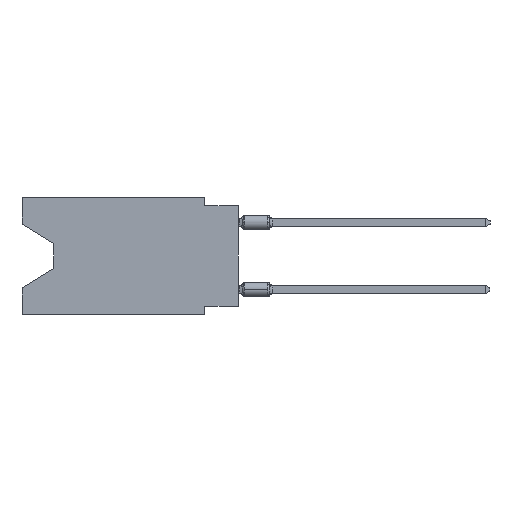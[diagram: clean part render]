
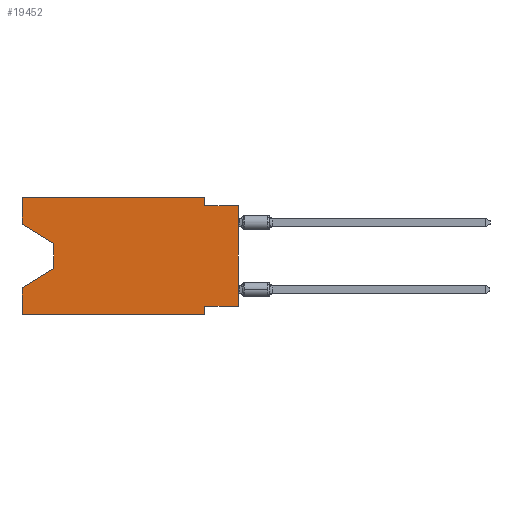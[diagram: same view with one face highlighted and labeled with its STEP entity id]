
A CAD part, left-side view. The second image highlights one B-rep face of the part: STEP entity #19452.
In plain terms, the highlighted planar face has unit normal (-1, 0, 0).
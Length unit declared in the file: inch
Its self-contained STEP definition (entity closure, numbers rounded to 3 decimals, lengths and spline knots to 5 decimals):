
#382 = VERTEX_POINT ( 'NONE', #17225 ) ;
#690 = EDGE_CURVE ( 'NONE', #25854, #382, #19527, .T. ) ;
#716 = CARTESIAN_POINT ( 'NONE',  ( 0., 0., -0.025 ) ) ;
#2037 = VERTEX_POINT ( 'NONE', #716 ) ;
#2414 = VERTEX_POINT ( 'NONE', #17462 ) ;
#3299 = CARTESIAN_POINT ( 'NONE',  ( 0., 0., 0. ) ) ;
#3395 = FACE_OUTER_BOUND ( 'NONE', #7323, .T. ) ;
#3515 = VECTOR ( 'NONE', #14902, 39.37008 ) ;
#3628 = CARTESIAN_POINT ( 'NONE',  ( 0., 0.1, -0.35 ) ) ;
#4466 = EDGE_CURVE ( 'NONE', #28183, #2037, #24819, .T. ) ;
#4566 = EDGE_CURVE ( 'NONE', #10817, #20446, #29086, .T. ) ;
#4943 = EDGE_CURVE ( 'NONE', #7981, #2414, #17398, .T. ) ;
#5505 = EDGE_CURVE ( 'NONE', #20446, #25854, #22928, .T. ) ;
#5774 = VERTEX_POINT ( 'NONE', #11917 ) ;
#6390 = ORIENTED_EDGE ( 'NONE', *, *, #4566, .T. ) ;
#6721 = CARTESIAN_POINT ( 'NONE',  ( 0., 0.645, -0.08025 ) ) ;
#7323 = EDGE_LOOP ( 'NONE', ( #6390, #21658, #12057, #11179, #10332, #13019, #8944, #12033, #10022, #23984, #8794, #13318 ) ) ;
#7707 = DIRECTION ( 'NONE',  ( 0., -1., 0. ) ) ;
#7981 = VERTEX_POINT ( 'NONE', #11597 ) ;
#8347 = LINE ( 'NONE', #3628, #17089 ) ;
#8558 = CARTESIAN_POINT ( 'NONE',  ( 0., 0.645, 0. ) ) ;
#8794 = ORIENTED_EDGE ( 'NONE', *, *, #20240, .F. ) ;
#8944 = ORIENTED_EDGE ( 'NONE', *, *, #9385, .F. ) ;
#9001 = AXIS2_PLACEMENT_3D ( 'NONE', #27774, #13300, #17863 ) ;
#9385 = EDGE_CURVE ( 'NONE', #28183, #25561, #27096, .T. ) ;
#9493 = EDGE_CURVE ( 'NONE', #28814, #5774, #28368, .T. ) ;
#10022 = ORIENTED_EDGE ( 'NONE', *, *, #28672, .F. ) ;
#10083 = DIRECTION ( 'NONE',  ( 0., -0.855, -0.519 ) ) ;
#10332 = ORIENTED_EDGE ( 'NONE', *, *, #9493, .T. ) ;
#10817 = VERTEX_POINT ( 'NONE', #6721 ) ;
#11179 = ORIENTED_EDGE ( 'NONE', *, *, #19741, .F. ) ;
#11256 = CARTESIAN_POINT ( 'NONE',  ( 0., 0.55, -0.212 ) ) ;
#11597 = CARTESIAN_POINT ( 'NONE',  ( 0., 0.1, 0. ) ) ;
#11917 = CARTESIAN_POINT ( 'NONE',  ( 0., 0.1, -0.35 ) ) ;
#12033 = ORIENTED_EDGE ( 'NONE', *, *, #4466, .T. ) ;
#12057 = ORIENTED_EDGE ( 'NONE', *, *, #690, .T. ) ;
#13019 = ORIENTED_EDGE ( 'NONE', *, *, #23464, .F. ) ;
#13300 = DIRECTION ( 'NONE',  ( 1., 0., 0. ) ) ;
#13318 = ORIENTED_EDGE ( 'NONE', *, *, #14769, .F. ) ;
#14384 = CARTESIAN_POINT ( 'NONE',  ( 0., 0.55, -0.212 ) ) ;
#14769 = EDGE_CURVE ( 'NONE', #10817, #29470, #20958, .T. ) ;
#14902 = DIRECTION ( 'NONE',  ( 0., 0., 1. ) ) ;
#14947 = VECTOR ( 'NONE', #7707, 39.37008 ) ;
#15029 = DIRECTION ( 'NONE',  ( 0., 0., -1. ) ) ;
#15297 = DIRECTION ( 'NONE',  ( 0., 1., 0. ) ) ;
#15713 = DIRECTION ( 'NONE',  ( 0., 0., -1. ) ) ;
#15815 = PLANE ( 'NONE',  #9001 ) ;
#15836 = VECTOR ( 'NONE', #26394, 39.37008 ) ;
#16535 = VECTOR ( 'NONE', #20327, 39.37008 ) ;
#17056 = CARTESIAN_POINT ( 'NONE',  ( 0., 0.645, 0. ) ) ;
#17089 = VECTOR ( 'NONE', #15713, 39.37008 ) ;
#17102 = VECTOR ( 'NONE', #10083, 39.37008 ) ;
#17225 = CARTESIAN_POINT ( 'NONE',  ( 0., 0.645, -0.26975 ) ) ;
#17398 = LINE ( 'NONE', #22275, #23680 ) ;
#17414 = CARTESIAN_POINT ( 'NONE',  ( 0., 0.1, -0.325 ) ) ;
#17462 = CARTESIAN_POINT ( 'NONE',  ( 0., 0.1, -0.025 ) ) ;
#17863 = DIRECTION ( 'NONE',  ( 0., 0., -1. ) ) ;
#18431 = CARTESIAN_POINT ( 'NONE',  ( 0., 0.55, -0.138 ) ) ;
#19251 = LINE ( 'NONE', #8558, #16535 ) ;
#19452 = ADVANCED_FACE ( 'NONE', ( #3395 ), #15815, .F. ) ;
#19527 = LINE ( 'NONE', #11256, #15836 ) ;
#19662 = LINE ( 'NONE', #29217, #14947 ) ;
#19741 = EDGE_CURVE ( 'NONE', #28814, #382, #24576, .T. ) ;
#19969 = CARTESIAN_POINT ( 'NONE',  ( 0., 0.645, -0.08025 ) ) ;
#20220 = CARTESIAN_POINT ( 'NONE',  ( 0., 0., -0.325 ) ) ;
#20240 = EDGE_CURVE ( 'NONE', #29470, #7981, #19251, .T. ) ;
#20327 = DIRECTION ( 'NONE',  ( 0., -1., 0. ) ) ;
#20446 = VERTEX_POINT ( 'NONE', #18431 ) ;
#20447 = CARTESIAN_POINT ( 'NONE',  ( 0., 0.55, -0.138 ) ) ;
#20958 = LINE ( 'NONE', #25802, #30195 ) ;
#21122 = DIRECTION ( 'NONE',  ( 0., 0., 1. ) ) ;
#21539 = VECTOR ( 'NONE', #24118, 39.37008 ) ;
#21658 = ORIENTED_EDGE ( 'NONE', *, *, #5505, .T. ) ;
#22275 = CARTESIAN_POINT ( 'NONE',  ( 0., 0.1, 0. ) ) ;
#22928 = LINE ( 'NONE', #20447, #27807 ) ;
#23241 = CARTESIAN_POINT ( 'NONE',  ( 0., 0.645, -0.35 ) ) ;
#23464 = EDGE_CURVE ( 'NONE', #25561, #5774, #8347, .T. ) ;
#23649 = CARTESIAN_POINT ( 'NONE',  ( 0., 0.645, -0.35 ) ) ;
#23680 = VECTOR ( 'NONE', #15029, 39.37008 ) ;
#23984 = ORIENTED_EDGE ( 'NONE', *, *, #4943, .F. ) ;
#24118 = DIRECTION ( 'NONE',  ( 0., 0., 1. ) ) ;
#24576 = LINE ( 'NONE', #17056, #21539 ) ;
#24819 = LINE ( 'NONE', #3299, #3515 ) ;
#25561 = VERTEX_POINT ( 'NONE', #17414 ) ;
#25802 = CARTESIAN_POINT ( 'NONE',  ( 0., 0.645, 0. ) ) ;
#25854 = VERTEX_POINT ( 'NONE', #14384 ) ;
#26394 = DIRECTION ( 'NONE',  ( 0., 0.855, -0.519 ) ) ;
#27096 = LINE ( 'NONE', #20220, #30553 ) ;
#27675 = DIRECTION ( 'NONE',  ( 0., 0., -1. ) ) ;
#27774 = CARTESIAN_POINT ( 'NONE',  ( 0., 0.645, 0. ) ) ;
#27807 = VECTOR ( 'NONE', #27675, 39.37008 ) ;
#28183 = VERTEX_POINT ( 'NONE', #28242 ) ;
#28242 = CARTESIAN_POINT ( 'NONE',  ( 0., 0., -0.325 ) ) ;
#28368 = LINE ( 'NONE', #23649, #29061 ) ;
#28672 = EDGE_CURVE ( 'NONE', #2414, #2037, #19662, .T. ) ;
#28814 = VERTEX_POINT ( 'NONE', #23241 ) ;
#29061 = VECTOR ( 'NONE', #30408, 39.37008 ) ;
#29086 = LINE ( 'NONE', #19969, #17102 ) ;
#29186 = CARTESIAN_POINT ( 'NONE',  ( 0., 0.645, 0. ) ) ;
#29217 = CARTESIAN_POINT ( 'NONE',  ( 0., 0., -0.025 ) ) ;
#29470 = VERTEX_POINT ( 'NONE', #29186 ) ;
#30195 = VECTOR ( 'NONE', #21122, 39.37008 ) ;
#30408 = DIRECTION ( 'NONE',  ( 0., -1., 0. ) ) ;
#30553 = VECTOR ( 'NONE', #15297, 39.37008 ) ;
